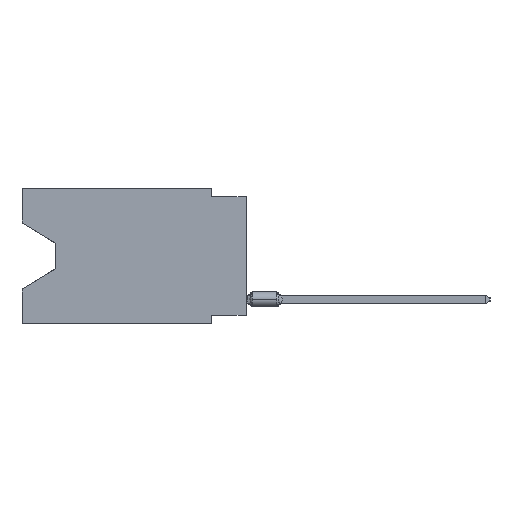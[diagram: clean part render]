
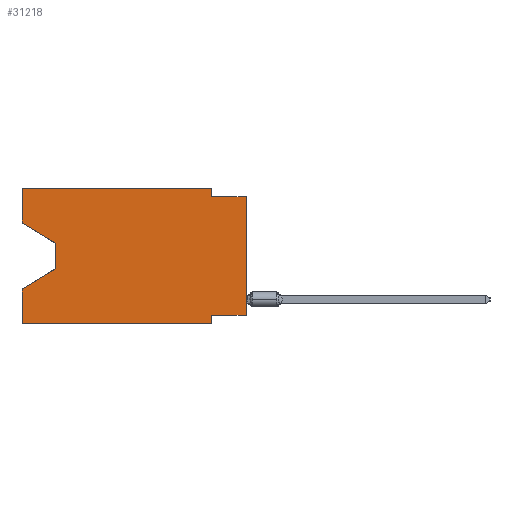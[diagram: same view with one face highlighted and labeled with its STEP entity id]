
A CAD part, left-side view. The second image highlights one B-rep face of the part: STEP entity #31218.
In plain terms, the highlighted planar face has unit normal (-1, 0, 0).
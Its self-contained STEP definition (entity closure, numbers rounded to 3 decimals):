
#44 = LINE ( 'NONE', #33355, #9930 ) ;
#282 = VECTOR ( 'NONE', #42252, 1000. ) ;
#288 = FACE_OUTER_BOUND ( 'NONE', #17821, .T. ) ;
#363 = DIRECTION ( 'NONE',  ( 0., -1., 0. ) ) ;
#843 = CARTESIAN_POINT ( 'NONE',  ( 0., 0., -0.635 ) ) ;
#1594 = EDGE_CURVE ( 'NONE', #44254, #21254, #4770, .T. ) ;
#2190 = VECTOR ( 'NONE', #4991, 1000. ) ;
#2580 = VECTOR ( 'NONE', #53002, 1000. ) ;
#2952 = CARTESIAN_POINT ( 'NONE',  ( 0., 16.383, -7.36 ) ) ;
#2991 = LINE ( 'NONE', #51977, #3757 ) ;
#3757 = VECTOR ( 'NONE', #36287, 1000. ) ;
#4306 = EDGE_CURVE ( 'NONE', #31307, #40363, #41761, .T. ) ;
#4770 = LINE ( 'NONE', #53133, #39577 ) ;
#4991 = DIRECTION ( 'NONE',  ( 0., 0., 1. ) ) ;
#5319 = DIRECTION ( 'NONE',  ( 0., 0., -1. ) ) ;
#5860 = DIRECTION ( 'NONE',  ( 0., -0.855, -0.519 ) ) ;
#6015 = ORIENTED_EDGE ( 'NONE', *, *, #10824, .F. ) ;
#6362 = LINE ( 'NONE', #20502, #52605 ) ;
#6958 = ORIENTED_EDGE ( 'NONE', *, *, #47322, .F. ) ;
#7521 = EDGE_CURVE ( 'NONE', #45584, #31307, #44, .T. ) ;
#8720 = CARTESIAN_POINT ( 'NONE',  ( 0., 2.54, -9.906 ) ) ;
#9266 = CARTESIAN_POINT ( 'NONE',  ( 0., 0., 0. ) ) ;
#9930 = VECTOR ( 'NONE', #19522, 1000. ) ;
#10700 = CARTESIAN_POINT ( 'NONE',  ( 0., 0., -9.271 ) ) ;
#10824 = EDGE_CURVE ( 'NONE', #58227, #32348, #32080, .T. ) ;
#12249 = AXIS2_PLACEMENT_3D ( 'NONE', #19455, #48328, #5319 ) ;
#12861 = CARTESIAN_POINT ( 'NONE',  ( 0., 13.97, -5.893 ) ) ;
#14078 = VECTOR ( 'NONE', #5860, 1000. ) ;
#15046 = PLANE ( 'NONE',  #12249 ) ;
#16883 = EDGE_CURVE ( 'NONE', #48892, #31394, #6362, .T. ) ;
#17821 = EDGE_LOOP ( 'NONE', ( #52153, #61963, #53228, #39044, #30672, #61564, #61285, #35679, #47687, #6015, #50472, #6958 ) ) ;
#19106 = EDGE_CURVE ( 'NONE', #31394, #21254, #50440, .T. ) ;
#19455 = CARTESIAN_POINT ( 'NONE',  ( 0., 16.383, 0. ) ) ;
#19522 = DIRECTION ( 'NONE',  ( 0., 0., -1. ) ) ;
#20502 = CARTESIAN_POINT ( 'NONE',  ( 0., 0., -9.271 ) ) ;
#20627 = LINE ( 'NONE', #49195, #14078 ) ;
#21254 = VERTEX_POINT ( 'NONE', #8720 ) ;
#23224 = DIRECTION ( 'NONE',  ( 0., 0.855, -0.519 ) ) ;
#25127 = EDGE_CURVE ( 'NONE', #58310, #58227, #44862, .T. ) ;
#25508 = CARTESIAN_POINT ( 'NONE',  ( 0., 0., -0.635 ) ) ;
#27872 = CARTESIAN_POINT ( 'NONE',  ( 0., 2.54, -9.271 ) ) ;
#30361 = DIRECTION ( 'NONE',  ( 0., 0., -1. ) ) ;
#30672 = ORIENTED_EDGE ( 'NONE', *, *, #1594, .T. ) ;
#30966 = CARTESIAN_POINT ( 'NONE',  ( 0., 16.383, -9.906 ) ) ;
#31218 = ADVANCED_FACE ( 'NONE', ( #288 ), #15046, .F. ) ;
#31307 = VERTEX_POINT ( 'NONE', #40765 ) ;
#31394 = VERTEX_POINT ( 'NONE', #27872 ) ;
#32023 = EDGE_CURVE ( 'NONE', #48892, #42609, #52294, .T. ) ;
#32080 = LINE ( 'NONE', #42132, #50313 ) ;
#32348 = VERTEX_POINT ( 'NONE', #55995 ) ;
#33205 = EDGE_CURVE ( 'NONE', #44254, #40363, #58363, .T. ) ;
#33355 = CARTESIAN_POINT ( 'NONE',  ( 0., 13.97, -4.013 ) ) ;
#35679 = ORIENTED_EDGE ( 'NONE', *, *, #32023, .T. ) ;
#35700 = VECTOR ( 'NONE', #30361, 1000. ) ;
#36287 = DIRECTION ( 'NONE',  ( 0., 0., 1. ) ) ;
#39044 = ORIENTED_EDGE ( 'NONE', *, *, #33205, .F. ) ;
#39577 = VECTOR ( 'NONE', #363, 1000. ) ;
#39856 = DIRECTION ( 'NONE',  ( 0., -1., 0. ) ) ;
#40363 = VERTEX_POINT ( 'NONE', #2952 ) ;
#40765 = CARTESIAN_POINT ( 'NONE',  ( 0., 13.97, -5.893 ) ) ;
#41327 = CARTESIAN_POINT ( 'NONE',  ( 0., 13.97, -4.013 ) ) ;
#41761 = LINE ( 'NONE', #12861, #41858 ) ;
#41858 = VECTOR ( 'NONE', #23224, 1000. ) ;
#42132 = CARTESIAN_POINT ( 'NONE',  ( 0., 2.54, 0. ) ) ;
#42252 = DIRECTION ( 'NONE',  ( 0., 0., 1. ) ) ;
#42609 = VERTEX_POINT ( 'NONE', #25508 ) ;
#44186 = LINE ( 'NONE', #843, #2580 ) ;
#44254 = VERTEX_POINT ( 'NONE', #30966 ) ;
#44562 = VERTEX_POINT ( 'NONE', #61717 ) ;
#44862 = LINE ( 'NONE', #58701, #55273 ) ;
#45421 = EDGE_CURVE ( 'NONE', #32348, #42609, #44186, .T. ) ;
#45584 = VERTEX_POINT ( 'NONE', #41327 ) ;
#47322 = EDGE_CURVE ( 'NONE', #44562, #58310, #2991, .T. ) ;
#47687 = ORIENTED_EDGE ( 'NONE', *, *, #45421, .F. ) ;
#48328 = DIRECTION ( 'NONE',  ( 1., 0., 0. ) ) ;
#48892 = VERTEX_POINT ( 'NONE', #10700 ) ;
#49195 = CARTESIAN_POINT ( 'NONE',  ( 0., 16.383, -2.546 ) ) ;
#49386 = DIRECTION ( 'NONE',  ( 0., 1., 0. ) ) ;
#49828 = CARTESIAN_POINT ( 'NONE',  ( 0., 2.54, -9.906 ) ) ;
#50313 = VECTOR ( 'NONE', #60975, 1000. ) ;
#50440 = LINE ( 'NONE', #49828, #35700 ) ;
#50472 = ORIENTED_EDGE ( 'NONE', *, *, #25127, .F. ) ;
#51977 = CARTESIAN_POINT ( 'NONE',  ( 0., 16.383, 0. ) ) ;
#52153 = ORIENTED_EDGE ( 'NONE', *, *, #52217, .T. ) ;
#52217 = EDGE_CURVE ( 'NONE', #44562, #45584, #20627, .T. ) ;
#52294 = LINE ( 'NONE', #9266, #282 ) ;
#52605 = VECTOR ( 'NONE', #49386, 1000. ) ;
#52923 = CARTESIAN_POINT ( 'NONE',  ( 0., 2.54, 0. ) ) ;
#53002 = DIRECTION ( 'NONE',  ( 0., -1., 0. ) ) ;
#53133 = CARTESIAN_POINT ( 'NONE',  ( 0., 16.383, -9.906 ) ) ;
#53228 = ORIENTED_EDGE ( 'NONE', *, *, #4306, .T. ) ;
#55273 = VECTOR ( 'NONE', #39856, 1000. ) ;
#55995 = CARTESIAN_POINT ( 'NONE',  ( 0., 2.54, -0.635 ) ) ;
#57745 = CARTESIAN_POINT ( 'NONE',  ( 0., 16.383, 0. ) ) ;
#58227 = VERTEX_POINT ( 'NONE', #52923 ) ;
#58310 = VERTEX_POINT ( 'NONE', #58558 ) ;
#58363 = LINE ( 'NONE', #57745, #2190 ) ;
#58558 = CARTESIAN_POINT ( 'NONE',  ( 0., 16.383, 0. ) ) ;
#58701 = CARTESIAN_POINT ( 'NONE',  ( 0., 16.383, 0. ) ) ;
#60975 = DIRECTION ( 'NONE',  ( 0., 0., -1. ) ) ;
#61285 = ORIENTED_EDGE ( 'NONE', *, *, #16883, .F. ) ;
#61564 = ORIENTED_EDGE ( 'NONE', *, *, #19106, .F. ) ;
#61717 = CARTESIAN_POINT ( 'NONE',  ( 0., 16.383, -2.546 ) ) ;
#61963 = ORIENTED_EDGE ( 'NONE', *, *, #7521, .T. ) ;
